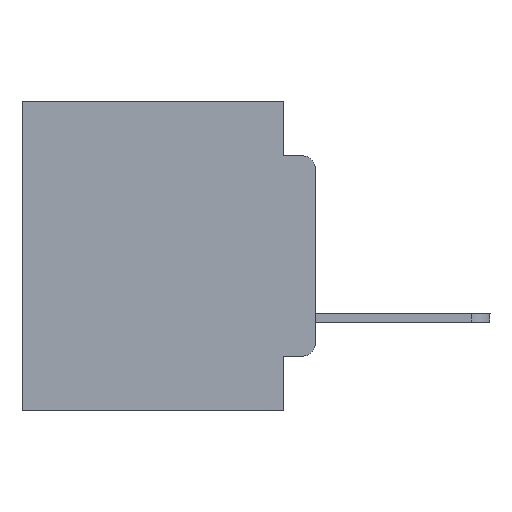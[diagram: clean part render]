
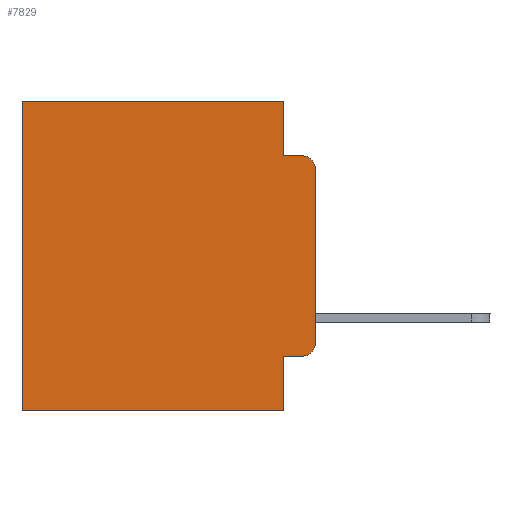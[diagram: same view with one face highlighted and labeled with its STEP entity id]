
A CAD part, left-side view. The second image highlights one B-rep face of the part: STEP entity #7829.
In plain terms, the highlighted planar face has unit normal (-1, 0, 0).
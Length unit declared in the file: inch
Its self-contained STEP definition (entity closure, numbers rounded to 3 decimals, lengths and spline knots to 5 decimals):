
#564 = CARTESIAN_POINT ( 'NONE',  ( 0.298, 0.02, -0.4115 ) ) ;
#1292 = VERTEX_POINT ( 'NONE', #24300 ) ;
#1394 = DIRECTION ( 'NONE',  ( 0., 0., -1. ) ) ;
#1632 = DIRECTION ( 'NONE',  ( 0., 1., 0. ) ) ;
#1972 = CARTESIAN_POINT ( 'NONE',  ( 0.298, 0.051, -0.4115 ) ) ;
#2265 = CARTESIAN_POINT ( 'NONE',  ( 0.298, 0.051, -0.0885 ) ) ;
#2388 = LINE ( 'NONE', #2265, #20137 ) ;
#2575 = ORIENTED_EDGE ( 'NONE', *, *, #6770, .F. ) ;
#3144 = EDGE_CURVE ( 'NONE', #11230, #9655, #8254, .T. ) ;
#4565 = VERTEX_POINT ( 'NONE', #18559 ) ;
#5597 = VERTEX_POINT ( 'NONE', #18812 ) ;
#5891 = CARTESIAN_POINT ( 'NONE',  ( 0.298, 0., -0.5 ) ) ;
#6300 = ORIENTED_EDGE ( 'NONE', *, *, #24503, .F. ) ;
#6331 = ORIENTED_EDGE ( 'NONE', *, *, #7170, .T. ) ;
#6439 = CIRCLE ( 'NONE', #6841, 0.02 ) ;
#6451 = EDGE_CURVE ( 'NONE', #11230, #5597, #25045, .T. ) ;
#6456 = CARTESIAN_POINT ( 'NONE',  ( 0.298, 0.051, -0.4115 ) ) ;
#6526 = EDGE_CURVE ( 'NONE', #23902, #19582, #13629, .T. ) ;
#6770 = EDGE_CURVE ( 'NONE', #11078, #4565, #18447, .T. ) ;
#6841 = AXIS2_PLACEMENT_3D ( 'NONE', #23089, #17683, #9348 ) ;
#6867 = DIRECTION ( 'NONE',  ( 0., 0., -1. ) ) ;
#6889 = DIRECTION ( 'NONE',  ( 0., 0., -1. ) ) ;
#7170 = EDGE_CURVE ( 'NONE', #15583, #25084, #18414, .T. ) ;
#7445 = CARTESIAN_POINT ( 'NONE',  ( 0.298, 0.051, 0. ) ) ;
#7461 = LINE ( 'NONE', #16844, #8642 ) ;
#7605 = CARTESIAN_POINT ( 'NONE',  ( 0.298, 0.051, -0.5 ) ) ;
#7829 = ADVANCED_FACE ( 'NONE', ( #19265 ), #13114, .F. ) ;
#8254 = LINE ( 'NONE', #16094, #19448 ) ;
#8642 = VECTOR ( 'NONE', #1394, 39.37008 ) ;
#9348 = DIRECTION ( 'NONE',  ( 0., 0., -1. ) ) ;
#9412 = DIRECTION ( 'NONE',  ( 0., 0., -1. ) ) ;
#9655 = VERTEX_POINT ( 'NONE', #21426 ) ;
#9717 = ORIENTED_EDGE ( 'NONE', *, *, #6451, .F. ) ;
#9772 = ORIENTED_EDGE ( 'NONE', *, *, #3144, .T. ) ;
#9783 = VECTOR ( 'NONE', #1632, 39.37008 ) ;
#10386 = ORIENTED_EDGE ( 'NONE', *, *, #18640, .T. ) ;
#10949 = ORIENTED_EDGE ( 'NONE', *, *, #15506, .T. ) ;
#11078 = VERTEX_POINT ( 'NONE', #22817 ) ;
#11230 = VERTEX_POINT ( 'NONE', #19983 ) ;
#11645 = CARTESIAN_POINT ( 'NONE',  ( 0.298, 0.473, -0.5 ) ) ;
#13114 = PLANE ( 'NONE',  #20989 ) ;
#13545 = DIRECTION ( 'NONE',  ( 0., 1., 0. ) ) ;
#13629 = LINE ( 'NONE', #5891, #9783 ) ;
#14707 = CARTESIAN_POINT ( 'NONE',  ( 0.298, 0.02, -0.3915 ) ) ;
#14985 = LINE ( 'NONE', #18974, #16047 ) ;
#15060 = CIRCLE ( 'NONE', #24911, 0.02 ) ;
#15506 = EDGE_CURVE ( 'NONE', #11078, #1292, #6439, .T. ) ;
#15583 = VERTEX_POINT ( 'NONE', #1972 ) ;
#15868 = EDGE_CURVE ( 'NONE', #25084, #4565, #15060, .T. ) ;
#16047 = VECTOR ( 'NONE', #6889, 39.37008 ) ;
#16094 = CARTESIAN_POINT ( 'NONE',  ( 0.298, 0., 0. ) ) ;
#16635 = DIRECTION ( 'NONE',  ( -1., 0., 0. ) ) ;
#16641 = CARTESIAN_POINT ( 'NONE',  ( 0.298, 0., 0. ) ) ;
#16844 = CARTESIAN_POINT ( 'NONE',  ( 0.298, 0.473, 0. ) ) ;
#17094 = DIRECTION ( 'NONE',  ( 0., 0., -1. ) ) ;
#17156 = ORIENTED_EDGE ( 'NONE', *, *, #6526, .F. ) ;
#17683 = DIRECTION ( 'NONE',  ( -1., 0., 0. ) ) ;
#17979 = DIRECTION ( 'NONE',  ( 0., -1., 0. ) ) ;
#18250 = VECTOR ( 'NONE', #20573, 39.37008 ) ;
#18414 = LINE ( 'NONE', #6456, #21100 ) ;
#18447 = LINE ( 'NONE', #16641, #19772 ) ;
#18559 = CARTESIAN_POINT ( 'NONE',  ( 0.298, 0., -0.3915 ) ) ;
#18640 = EDGE_CURVE ( 'NONE', #9655, #19582, #7461, .T. ) ;
#18661 = DIRECTION ( 'NONE',  ( 0., -1., 0. ) ) ;
#18812 = CARTESIAN_POINT ( 'NONE',  ( 0.298, 0.051, -0.0885 ) ) ;
#18974 = CARTESIAN_POINT ( 'NONE',  ( 0.298, 0.051, 0. ) ) ;
#19255 = ORIENTED_EDGE ( 'NONE', *, *, #19514, .F. ) ;
#19265 = FACE_OUTER_BOUND ( 'NONE', #23469, .T. ) ;
#19448 = VECTOR ( 'NONE', #13545, 39.37008 ) ;
#19514 = EDGE_CURVE ( 'NONE', #15583, #23902, #14985, .T. ) ;
#19582 = VERTEX_POINT ( 'NONE', #11645 ) ;
#19772 = VECTOR ( 'NONE', #6867, 39.37008 ) ;
#19983 = CARTESIAN_POINT ( 'NONE',  ( 0.298, 0.051, 0. ) ) ;
#20137 = VECTOR ( 'NONE', #17979, 39.37008 ) ;
#20573 = DIRECTION ( 'NONE',  ( 0., 0., -1. ) ) ;
#20952 = DIRECTION ( 'NONE',  ( 1., 0., 0. ) ) ;
#20989 = AXIS2_PLACEMENT_3D ( 'NONE', #24536, #20952, #17094 ) ;
#21100 = VECTOR ( 'NONE', #18661, 39.37008 ) ;
#21426 = CARTESIAN_POINT ( 'NONE',  ( 0.298, 0.473, 0. ) ) ;
#22817 = CARTESIAN_POINT ( 'NONE',  ( 0.298, 0., -0.1085 ) ) ;
#23089 = CARTESIAN_POINT ( 'NONE',  ( 0.298, 0.02, -0.1085 ) ) ;
#23469 = EDGE_LOOP ( 'NONE', ( #2575, #10949, #6300, #9717, #9772, #10386, #17156, #19255, #6331, #24374 ) ) ;
#23902 = VERTEX_POINT ( 'NONE', #7605 ) ;
#24300 = CARTESIAN_POINT ( 'NONE',  ( 0.298, 0.02, -0.0885 ) ) ;
#24374 = ORIENTED_EDGE ( 'NONE', *, *, #15868, .T. ) ;
#24503 = EDGE_CURVE ( 'NONE', #5597, #1292, #2388, .T. ) ;
#24536 = CARTESIAN_POINT ( 'NONE',  ( 0.298, 0., 0. ) ) ;
#24911 = AXIS2_PLACEMENT_3D ( 'NONE', #14707, #16635, #9412 ) ;
#25045 = LINE ( 'NONE', #7445, #18250 ) ;
#25084 = VERTEX_POINT ( 'NONE', #564 ) ;
